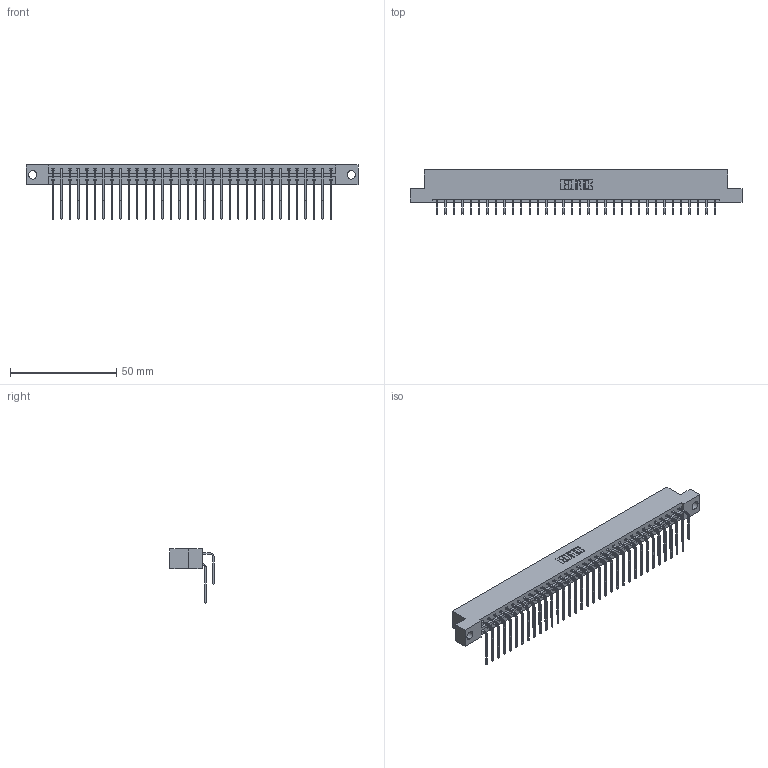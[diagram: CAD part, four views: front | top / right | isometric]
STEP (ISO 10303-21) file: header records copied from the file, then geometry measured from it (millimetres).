
FILE_DESCRIPTION (( 'STEP AP203' ), '1' );
FILE_NAME ('833-068-559-204.STEP', '2020-06-05T11:27:16', ( '' ), ( '' ), 'SwSTEP 2.0', 'SolidWorks 2020', '' );
FILE_SCHEMA (( 'CONFIG_CONTROL_DESIGN' ));
Length unit declared in the file: inch
Products named in the file (4): 833-068-559-204; 345-292-001_558 559 Tail - 1; 345-292-001_559 Tail - 2; 833 Part_Flush - .156 Dia - TH
Assembly tree (69 placements, depth 2):
  833-068-559-204
    833 Part_Flush - .156 Dia - TH
    345-292-001_558 559 Tail - 1  x34
    345-292-001_559 Tail - 2  x34
Bounding box: 156.26 x 20.9 x 25.53 mm (x, y, z)
Volume: 16182.9 mm3; surface area: 20799.7 mm2
Topology: 69 solids, 69 shells, 3786 faces, 11259 edges, 7414 vertices
Faces by surface type: plane 2654, cylinder 1132
Entity records: 24695 total; most frequent: CARTESIAN_POINT 4153, ORIENTED_EDGE 4038, DIRECTION 3543, EDGE_CURVE 2019, LINE 1851, VECTOR 1851, VERTEX_POINT 1342, AXIS2_PLACEMENT_3D 846
